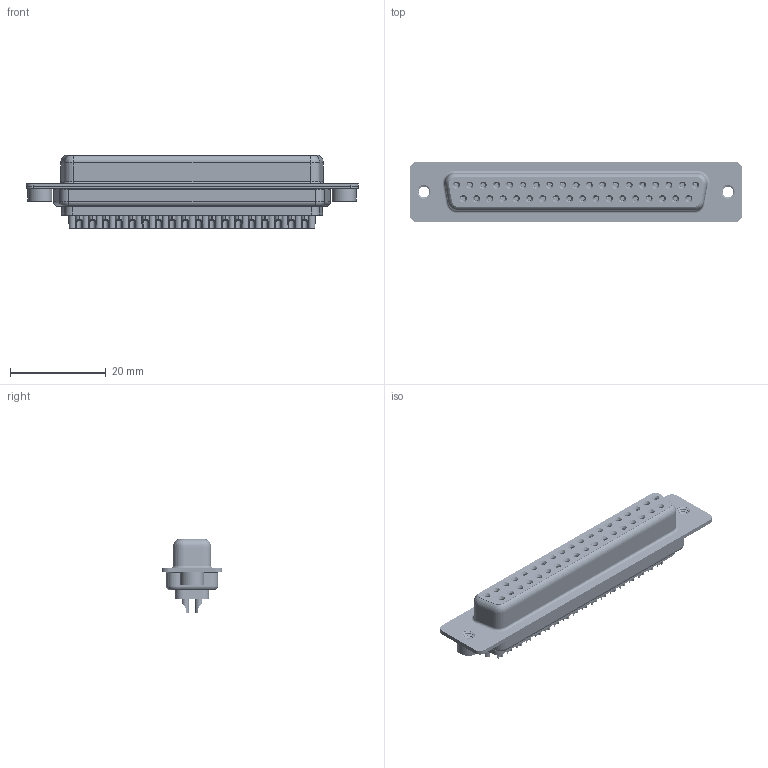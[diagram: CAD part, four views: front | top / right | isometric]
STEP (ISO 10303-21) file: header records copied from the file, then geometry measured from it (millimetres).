
FILE_DESCRIPTION (( 'STEP AP203' ), '1' );
FILE_NAME ('628-037-622-542.STEP', '2018-10-20T05:20:22', ( '' ), ( '' ), 'SwSTEP 2.0', 'SolidWorks 2016', '' );
FILE_SCHEMA (( 'CONFIG_CONTROL_DESIGN' ));
Length unit declared in the file: millimetre
Products named in the file (7): 628-037-622-542; 628 Housing_37 LP; 628 Shell Front_37 Contacts; 628 Shell Rear_37 Contacts; 628 Contact Row 1_22L; 628 Contact Row 2_22L; 628 4-40 Threaded Rivet
Assembly tree (42 placements, depth 2):
  628-037-622-542
    628 Housing_37 LP
    628 Shell Front_37 Contacts
    628 Shell Rear_37 Contacts
    628 Contact Row 1_22L  x19
    628 Contact Row 2_22L  x18
    628 4-40 Threaded Rivet  x2
Bounding box: 69.3 x 12.6 x 15.35 mm (x, y, z)
Volume: 5819.3 mm3; surface area: 13684.3 mm2
Topology: 42 solids, 42 shells, 3545 faces, 8982 edges, 5644 vertices
Faces by surface type: cylinder 1049, plane 841, bspline 746, torus 718, cone 191
Entity records: 29395 total; most frequent: CARTESIAN_POINT 7661, DIRECTION 4508, ORIENTED_EDGE 3940, EDGE_CURVE 1970, AXIS2_PLACEMENT_3D 1902, VERTEX_POINT 1251, EDGE_LOOP 1059, CIRCLE 1048
